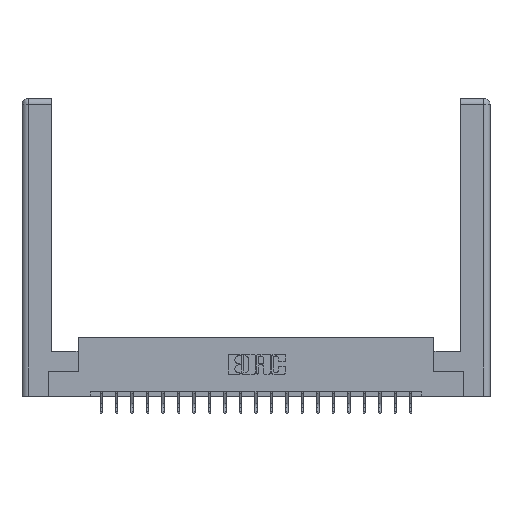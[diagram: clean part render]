
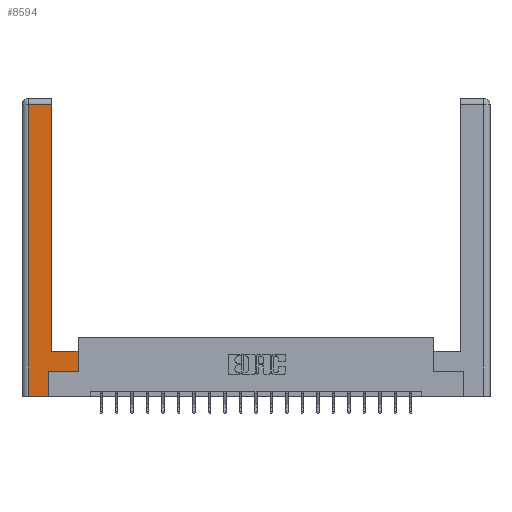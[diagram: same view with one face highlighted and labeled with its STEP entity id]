
A CAD part, top view. The second image highlights one B-rep face of the part: STEP entity #8594.
In plain terms, the highlighted planar face has unit normal (0, 0, 1).
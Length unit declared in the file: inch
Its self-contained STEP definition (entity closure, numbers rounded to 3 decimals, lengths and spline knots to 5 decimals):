
#66 = DIRECTION ( 'NONE',  ( -1., 0., 0. ) ) ;
#977 = DIRECTION ( 'NONE',  ( 1., 0., 0. ) ) ;
#2054 = DIRECTION ( 'NONE',  ( 0., 1., 0. ) ) ;
#2102 = EDGE_CURVE ( 'NONE', #12259, #21659, #18352, .T. ) ;
#2139 = EDGE_CURVE ( 'NONE', #19270, #8244, #13096, .T. ) ;
#2387 = DIRECTION ( 'NONE',  ( 0., -1., 0. ) ) ;
#3419 = CARTESIAN_POINT ( 'NONE',  ( 0.0615, 2.94, 0. ) ) ;
#4379 = LINE ( 'NONE', #16246, #16772 ) ;
#4510 = FACE_OUTER_BOUND ( 'NONE', #19206, .T. ) ;
#4675 = DIRECTION ( 'NONE',  ( 0., 1., 0. ) ) ;
#4854 = LINE ( 'NONE', #10189, #19338 ) ;
#4970 = DIRECTION ( 'NONE',  ( -1., 0., 0. ) ) ;
#5209 = CARTESIAN_POINT ( 'NONE',  ( 0.295, 2.94, 0. ) ) ;
#6883 = ORIENTED_EDGE ( 'NONE', *, *, #19805, .T. ) ;
#6913 = CARTESIAN_POINT ( 'NONE',  ( 0.565, 0.245, 0. ) ) ;
#7498 = CARTESIAN_POINT ( 'NONE',  ( 0.565, 0.45, 0. ) ) ;
#7688 = ORIENTED_EDGE ( 'NONE', *, *, #8852, .T. ) ;
#7940 = CARTESIAN_POINT ( 'NONE',  ( 0.0615, 0., 0. ) ) ;
#8183 = LINE ( 'NONE', #15414, #11089 ) ;
#8196 = VECTOR ( 'NONE', #2387, 39.37008 ) ;
#8244 = VERTEX_POINT ( 'NONE', #21542 ) ;
#8432 = CARTESIAN_POINT ( 'NONE',  ( 0.295, 0.45, 0. ) ) ;
#8594 = ADVANCED_FACE ( 'NONE', ( #4510 ), #10316, .F. ) ;
#8852 = EDGE_CURVE ( 'NONE', #21659, #19155, #8183, .T. ) ;
#9858 = VERTEX_POINT ( 'NONE', #6913 ) ;
#9981 = DIRECTION ( 'NONE',  ( -1., 0., 0. ) ) ;
#10031 = LINE ( 'NONE', #15818, #8196 ) ;
#10179 = DIRECTION ( 'NONE',  ( 0., 0., -1. ) ) ;
#10189 = CARTESIAN_POINT ( 'NONE',  ( 0.295, 0.45, 0. ) ) ;
#10316 = PLANE ( 'NONE',  #16353 ) ;
#10445 = VECTOR ( 'NONE', #9981, 39.37008 ) ;
#11089 = VECTOR ( 'NONE', #2054, 39.37008 ) ;
#11201 = ORIENTED_EDGE ( 'NONE', *, *, #2139, .T. ) ;
#12254 = CARTESIAN_POINT ( 'NONE',  ( 0.565, 0.45, 0. ) ) ;
#12259 = VERTEX_POINT ( 'NONE', #7940 ) ;
#13096 = LINE ( 'NONE', #3419, #10445 ) ;
#13441 = CARTESIAN_POINT ( 'NONE',  ( 0., 0., 0. ) ) ;
#13721 = CARTESIAN_POINT ( 'NONE',  ( 0.265, 0.245, 0. ) ) ;
#13848 = EDGE_CURVE ( 'NONE', #19155, #9858, #19870, .T. ) ;
#13881 = LINE ( 'NONE', #12254, #14658 ) ;
#13900 = VECTOR ( 'NONE', #14960, 39.37008 ) ;
#14029 = DIRECTION ( 'NONE',  ( 0., 1., 0. ) ) ;
#14239 = ORIENTED_EDGE ( 'NONE', *, *, #13848, .T. ) ;
#14505 = ORIENTED_EDGE ( 'NONE', *, *, #16492, .T. ) ;
#14650 = VECTOR ( 'NONE', #977, 39.37008 ) ;
#14658 = VECTOR ( 'NONE', #14029, 39.37008 ) ;
#14960 = DIRECTION ( 'NONE',  ( 1., 0., 0. ) ) ;
#15414 = CARTESIAN_POINT ( 'NONE',  ( 0.265, 0.245, 0. ) ) ;
#15818 = CARTESIAN_POINT ( 'NONE',  ( 0.0615, 0., 0. ) ) ;
#16161 = CARTESIAN_POINT ( 'NONE',  ( 0.265, 0., 0. ) ) ;
#16246 = CARTESIAN_POINT ( 'NONE',  ( 0.295, 3., 0. ) ) ;
#16353 = AXIS2_PLACEMENT_3D ( 'NONE', #13441, #10179, #66 ) ;
#16492 = EDGE_CURVE ( 'NONE', #8244, #12259, #10031, .T. ) ;
#16772 = VECTOR ( 'NONE', #4675, 39.37008 ) ;
#16842 = CARTESIAN_POINT ( 'NONE',  ( 0.265, 0., 0. ) ) ;
#18111 = VERTEX_POINT ( 'NONE', #8432 ) ;
#18352 = LINE ( 'NONE', #16842, #13900 ) ;
#18490 = ORIENTED_EDGE ( 'NONE', *, *, #18593, .T. ) ;
#18593 = EDGE_CURVE ( 'NONE', #18111, #19270, #4379, .T. ) ;
#18785 = ORIENTED_EDGE ( 'NONE', *, *, #19013, .T. ) ;
#19013 = EDGE_CURVE ( 'NONE', #9858, #21094, #13881, .T. ) ;
#19155 = VERTEX_POINT ( 'NONE', #13721 ) ;
#19206 = EDGE_LOOP ( 'NONE', ( #18490, #11201, #14505, #21389, #7688, #14239, #18785, #6883 ) ) ;
#19270 = VERTEX_POINT ( 'NONE', #5209 ) ;
#19338 = VECTOR ( 'NONE', #4970, 39.37008 ) ;
#19805 = EDGE_CURVE ( 'NONE', #21094, #18111, #4854, .T. ) ;
#19870 = LINE ( 'NONE', #21333, #14650 ) ;
#21094 = VERTEX_POINT ( 'NONE', #7498 ) ;
#21333 = CARTESIAN_POINT ( 'NONE',  ( 0.565, 0.245, 0. ) ) ;
#21389 = ORIENTED_EDGE ( 'NONE', *, *, #2102, .T. ) ;
#21542 = CARTESIAN_POINT ( 'NONE',  ( 0.0615, 2.94, 0. ) ) ;
#21659 = VERTEX_POINT ( 'NONE', #16161 ) ;
